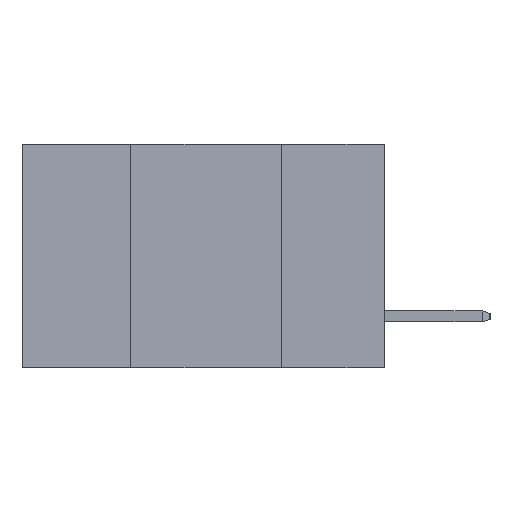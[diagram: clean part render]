
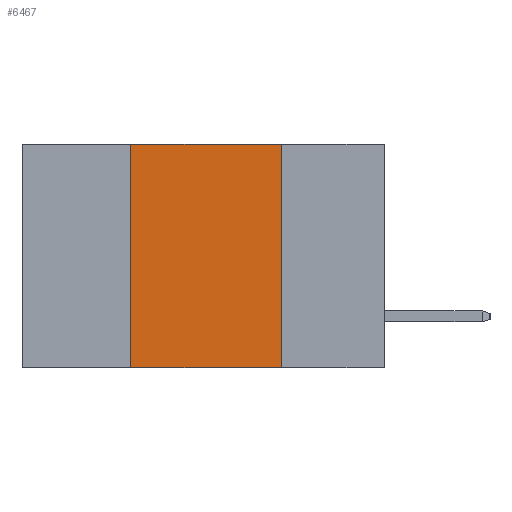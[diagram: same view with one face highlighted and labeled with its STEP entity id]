
A CAD part, left-side view. The second image highlights one B-rep face of the part: STEP entity #6467.
In plain terms, the highlighted planar face has unit normal (-1, 0, 0).
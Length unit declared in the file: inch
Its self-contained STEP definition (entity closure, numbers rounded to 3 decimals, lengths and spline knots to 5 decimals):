
#18 = VERTEX_POINT ( 'NONE', #10534 ) ;
#244 = VERTEX_POINT ( 'NONE', #9479 ) ;
#512 = ORIENTED_EDGE ( 'NONE', *, *, #5790, .F. ) ;
#894 = DIRECTION ( 'NONE',  ( 0., 0., 1. ) ) ;
#1071 = CARTESIAN_POINT ( 'NONE',  ( 0., 0.17, 0. ) ) ;
#1501 = CARTESIAN_POINT ( 'NONE',  ( 0., 0.6, 0. ) ) ;
#1967 = CARTESIAN_POINT ( 'NONE',  ( 0., 0.17, 0. ) ) ;
#3383 = LINE ( 'NONE', #1501, #9758 ) ;
#3895 = VECTOR ( 'NONE', #5005, 39.37008 ) ;
#5005 = DIRECTION ( 'NONE',  ( 0., 0., -1. ) ) ;
#5468 = VECTOR ( 'NONE', #894, 39.37008 ) ;
#5536 = LINE ( 'NONE', #7856, #7413 ) ;
#5642 = ORIENTED_EDGE ( 'NONE', *, *, #9274, .T. ) ;
#5692 = ORIENTED_EDGE ( 'NONE', *, *, #5755, .F. ) ;
#5755 = EDGE_CURVE ( 'NONE', #7699, #244, #8209, .T. ) ;
#5790 = EDGE_CURVE ( 'NONE', #8155, #7699, #3383, .T. ) ;
#5951 = EDGE_CURVE ( 'NONE', #18, #8155, #7588, .T. ) ;
#6026 = DIRECTION ( 'NONE',  ( 0., -1., 0. ) ) ;
#6467 = ADVANCED_FACE ( 'NONE', ( #7715 ), #9630, .F. ) ;
#6743 = CARTESIAN_POINT ( 'NONE',  ( 0., 0.42, 0. ) ) ;
#7187 = ORIENTED_EDGE ( 'NONE', *, *, #5951, .F. ) ;
#7285 = CARTESIAN_POINT ( 'NONE',  ( 0., 0.42, 0. ) ) ;
#7294 = AXIS2_PLACEMENT_3D ( 'NONE', #9588, #9450, #9442 ) ;
#7413 = VECTOR ( 'NONE', #6026, 39.37008 ) ;
#7588 = LINE ( 'NONE', #6743, #5468 ) ;
#7699 = VERTEX_POINT ( 'NONE', #1071 ) ;
#7715 = FACE_OUTER_BOUND ( 'NONE', #8144, .T. ) ;
#7856 = CARTESIAN_POINT ( 'NONE',  ( 0., 0.6, -0.37 ) ) ;
#8144 = EDGE_LOOP ( 'NONE', ( #5692, #512, #7187, #5642 ) ) ;
#8155 = VERTEX_POINT ( 'NONE', #7285 ) ;
#8209 = LINE ( 'NONE', #1967, #3895 ) ;
#9274 = EDGE_CURVE ( 'NONE', #18, #244, #5536, .T. ) ;
#9442 = DIRECTION ( 'NONE',  ( 0., 0., -1. ) ) ;
#9450 = DIRECTION ( 'NONE',  ( 1., 0., 0. ) ) ;
#9479 = CARTESIAN_POINT ( 'NONE',  ( 0., 0.17, -0.37 ) ) ;
#9588 = CARTESIAN_POINT ( 'NONE',  ( 0., 0.6, 0. ) ) ;
#9630 = PLANE ( 'NONE',  #7294 ) ;
#9758 = VECTOR ( 'NONE', #10378, 39.37008 ) ;
#10378 = DIRECTION ( 'NONE',  ( 0., -1., 0. ) ) ;
#10534 = CARTESIAN_POINT ( 'NONE',  ( 0., 0.42, -0.37 ) ) ;
